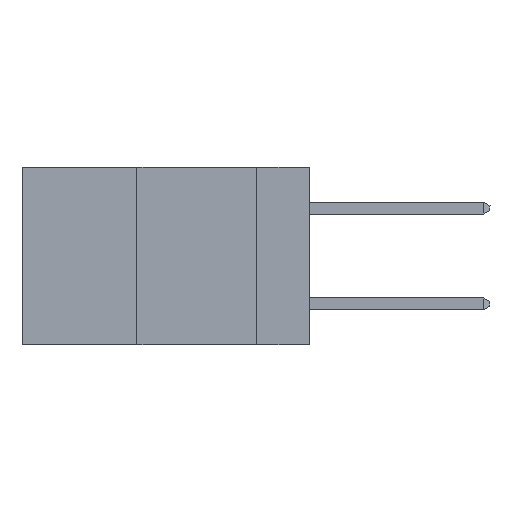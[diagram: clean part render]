
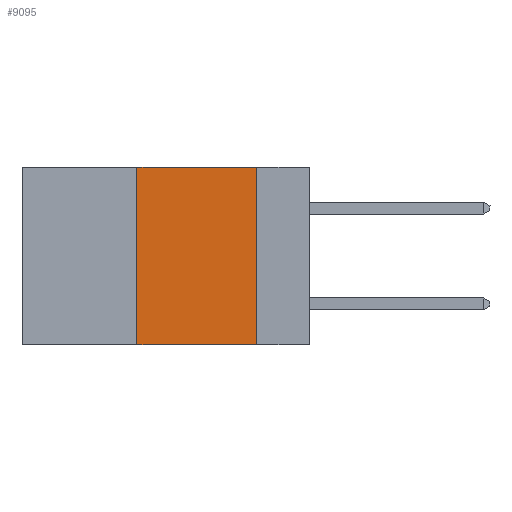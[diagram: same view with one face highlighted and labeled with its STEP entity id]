
A CAD part, left-side view. The second image highlights one B-rep face of the part: STEP entity #9095.
In plain terms, the highlighted planar face has unit normal (-1, 0, 0).
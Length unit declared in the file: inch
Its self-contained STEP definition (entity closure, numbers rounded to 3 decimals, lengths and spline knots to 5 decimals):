
#872 = VECTOR ( 'NONE', #9305, 39.37008 ) ;
#978 = EDGE_CURVE ( 'NONE', #6322, #2126, #12200, .T. ) ;
#1376 = VERTEX_POINT ( 'NONE', #1380 ) ;
#1380 = CARTESIAN_POINT ( 'NONE',  ( 0., 0.11, 0. ) ) ;
#1769 = CARTESIAN_POINT ( 'NONE',  ( 0., 0.36, 0. ) ) ;
#1882 = CARTESIAN_POINT ( 'NONE',  ( 0., 0.11, -0.37 ) ) ;
#2126 = VERTEX_POINT ( 'NONE', #1769 ) ;
#2483 = VECTOR ( 'NONE', #2983, 39.37008 ) ;
#2626 = VERTEX_POINT ( 'NONE', #1882 ) ;
#2812 = ORIENTED_EDGE ( 'NONE', *, *, #11222, .T. ) ;
#2818 = AXIS2_PLACEMENT_3D ( 'NONE', #7141, #6233, #7268 ) ;
#2983 = DIRECTION ( 'NONE',  ( 0., -1., 0. ) ) ;
#3527 = CARTESIAN_POINT ( 'NONE',  ( 0., 0.6, 0. ) ) ;
#4562 = LINE ( 'NONE', #3527, #11496 ) ;
#5332 = DIRECTION ( 'NONE',  ( 0., 0., -1. ) ) ;
#5723 = ORIENTED_EDGE ( 'NONE', *, *, #10170, .F. ) ;
#6233 = DIRECTION ( 'NONE',  ( 1., 0., 0. ) ) ;
#6322 = VERTEX_POINT ( 'NONE', #7406 ) ;
#6956 = LINE ( 'NONE', #10898, #2483 ) ;
#7141 = CARTESIAN_POINT ( 'NONE',  ( 0., 0.6, 0. ) ) ;
#7205 = LINE ( 'NONE', #12230, #10923 ) ;
#7268 = DIRECTION ( 'NONE',  ( 0., 0., -1. ) ) ;
#7406 = CARTESIAN_POINT ( 'NONE',  ( 0., 0.36, -0.37 ) ) ;
#8291 = PLANE ( 'NONE',  #2818 ) ;
#8297 = EDGE_LOOP ( 'NONE', ( #9635, #5723, #9831, #2812 ) ) ;
#9095 = ADVANCED_FACE ( 'NONE', ( #11139 ), #8291, .F. ) ;
#9305 = DIRECTION ( 'NONE',  ( 0., 0., 1. ) ) ;
#9635 = ORIENTED_EDGE ( 'NONE', *, *, #11350, .F. ) ;
#9831 = ORIENTED_EDGE ( 'NONE', *, *, #978, .F. ) ;
#10170 = EDGE_CURVE ( 'NONE', #2126, #1376, #4562, .T. ) ;
#10898 = CARTESIAN_POINT ( 'NONE',  ( 0., 0.6, -0.37 ) ) ;
#10923 = VECTOR ( 'NONE', #5332, 39.37008 ) ;
#11118 = CARTESIAN_POINT ( 'NONE',  ( 0., 0.36, 0. ) ) ;
#11139 = FACE_OUTER_BOUND ( 'NONE', #8297, .T. ) ;
#11222 = EDGE_CURVE ( 'NONE', #6322, #2626, #6956, .T. ) ;
#11350 = EDGE_CURVE ( 'NONE', #1376, #2626, #7205, .T. ) ;
#11496 = VECTOR ( 'NONE', #12485, 39.37008 ) ;
#12200 = LINE ( 'NONE', #11118, #872 ) ;
#12230 = CARTESIAN_POINT ( 'NONE',  ( 0., 0.11, 0. ) ) ;
#12485 = DIRECTION ( 'NONE',  ( 0., -1., 0. ) ) ;
